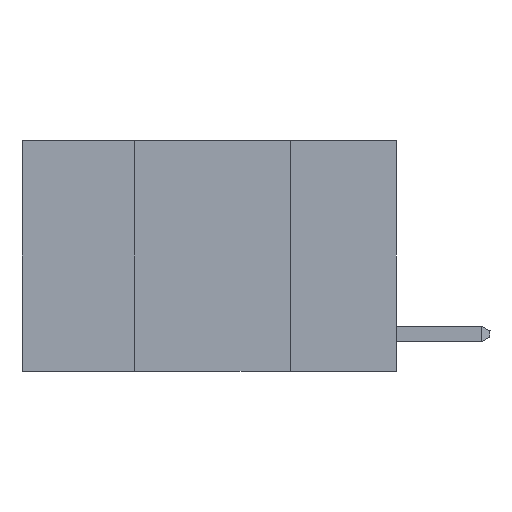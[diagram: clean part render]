
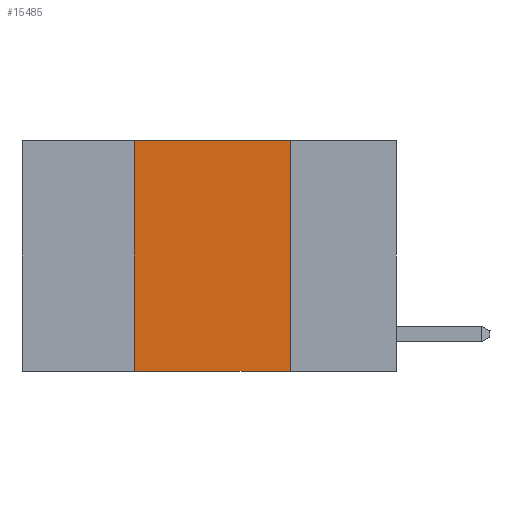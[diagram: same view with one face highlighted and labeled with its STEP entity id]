
A CAD part, left-side view. The second image highlights one B-rep face of the part: STEP entity #15485.
In plain terms, the highlighted planar face has unit normal (-1, 0, 0).
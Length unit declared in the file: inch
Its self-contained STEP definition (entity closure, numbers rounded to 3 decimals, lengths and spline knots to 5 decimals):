
#766 = LINE ( 'NONE', #19962, #17977 ) ;
#1188 = CARTESIAN_POINT ( 'NONE',  ( 0., 0.42, -0.37 ) ) ;
#1330 = DIRECTION ( 'NONE',  ( 0., 0., 1. ) ) ;
#1480 = ORIENTED_EDGE ( 'NONE', *, *, #3572, .T. ) ;
#1482 = LINE ( 'NONE', #11801, #25618 ) ;
#2476 = DIRECTION ( 'NONE',  ( 0., 0., -1. ) ) ;
#3572 = EDGE_CURVE ( 'NONE', #14884, #27243, #18502, .T. ) ;
#5740 = EDGE_CURVE ( 'NONE', #23875, #27243, #1482, .T. ) ;
#5906 = AXIS2_PLACEMENT_3D ( 'NONE', #24354, #26714, #12765 ) ;
#7229 = CARTESIAN_POINT ( 'NONE',  ( 0., 0.17, 0. ) ) ;
#8088 = PLANE ( 'NONE',  #5906 ) ;
#8743 = FACE_OUTER_BOUND ( 'NONE', #29760, .T. ) ;
#9418 = EDGE_CURVE ( 'NONE', #15521, #23875, #22640, .T. ) ;
#9679 = DIRECTION ( 'NONE',  ( 0., -1., 0. ) ) ;
#11576 = VECTOR ( 'NONE', #11618, 39.37008 ) ;
#11618 = DIRECTION ( 'NONE',  ( 0., -1., 0. ) ) ;
#11801 = CARTESIAN_POINT ( 'NONE',  ( 0., 0.17, 0. ) ) ;
#12765 = DIRECTION ( 'NONE',  ( 0., 0., -1. ) ) ;
#14884 = VERTEX_POINT ( 'NONE', #1188 ) ;
#15029 = CARTESIAN_POINT ( 'NONE',  ( 0., 0.17, -0.37 ) ) ;
#15485 = ADVANCED_FACE ( 'NONE', ( #8743 ), #8088, .F. ) ;
#15521 = VERTEX_POINT ( 'NONE', #24458 ) ;
#16428 = VECTOR ( 'NONE', #9679, 39.37008 ) ;
#17222 = ORIENTED_EDGE ( 'NONE', *, *, #9418, .F. ) ;
#17977 = VECTOR ( 'NONE', #1330, 39.37008 ) ;
#18502 = LINE ( 'NONE', #20899, #11576 ) ;
#19962 = CARTESIAN_POINT ( 'NONE',  ( 0., 0.42, 0. ) ) ;
#20899 = CARTESIAN_POINT ( 'NONE',  ( 0., 0.6, -0.37 ) ) ;
#21379 = EDGE_CURVE ( 'NONE', #14884, #15521, #766, .T. ) ;
#22640 = LINE ( 'NONE', #25954, #16428 ) ;
#23875 = VERTEX_POINT ( 'NONE', #7229 ) ;
#24354 = CARTESIAN_POINT ( 'NONE',  ( 0., 0.6, 0. ) ) ;
#24458 = CARTESIAN_POINT ( 'NONE',  ( 0., 0.42, 0. ) ) ;
#25614 = ORIENTED_EDGE ( 'NONE', *, *, #21379, .F. ) ;
#25618 = VECTOR ( 'NONE', #2476, 39.37008 ) ;
#25954 = CARTESIAN_POINT ( 'NONE',  ( 0., 0.6, 0. ) ) ;
#26704 = ORIENTED_EDGE ( 'NONE', *, *, #5740, .F. ) ;
#26714 = DIRECTION ( 'NONE',  ( 1., 0., 0. ) ) ;
#27243 = VERTEX_POINT ( 'NONE', #15029 ) ;
#29760 = EDGE_LOOP ( 'NONE', ( #26704, #17222, #25614, #1480 ) ) ;
